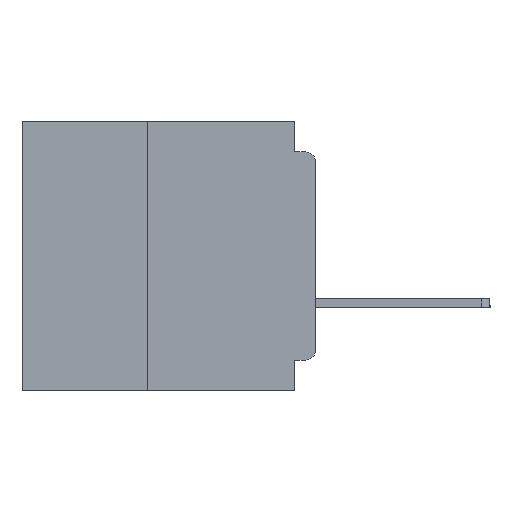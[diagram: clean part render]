
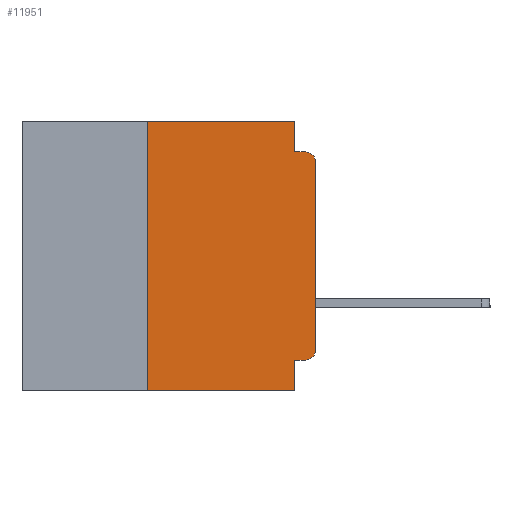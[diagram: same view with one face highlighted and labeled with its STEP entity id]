
A CAD part, left-side view. The second image highlights one B-rep face of the part: STEP entity #11951.
In plain terms, the highlighted planar face has unit normal (-1, 0, 0).
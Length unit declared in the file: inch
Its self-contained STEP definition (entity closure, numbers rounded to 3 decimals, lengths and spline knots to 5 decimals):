
#849 = PLANE ( 'NONE',  #15594 ) ;
#1895 = VERTEX_POINT ( 'NONE', #27323 ) ;
#2521 = ORIENTED_EDGE ( 'NONE', *, *, #34587, .F. ) ;
#2695 = LINE ( 'NONE', #43470, #38850 ) ;
#3022 = CARTESIAN_POINT ( 'NONE',  ( 0., 0.437, 0. ) ) ;
#3122 = EDGE_CURVE ( 'NONE', #5375, #38927, #2695, .T. ) ;
#3752 = ORIENTED_EDGE ( 'NONE', *, *, #7106, .F. ) ;
#3895 = CARTESIAN_POINT ( 'NONE',  ( 0., 0.25, -0.4 ) ) ;
#4044 = DIRECTION ( 'NONE',  ( 0., -1., 0. ) ) ;
#4057 = VERTEX_POINT ( 'NONE', #22687 ) ;
#4063 = DIRECTION ( 'NONE',  ( 0., -1., 0. ) ) ;
#4411 = DIRECTION ( 'NONE',  ( 0., 0., -1. ) ) ;
#5375 = VERTEX_POINT ( 'NONE', #37397 ) ;
#6188 = VECTOR ( 'NONE', #28904, 39.37008 ) ;
#6749 = CIRCLE ( 'NONE', #36059, 0.015 ) ;
#7106 = EDGE_CURVE ( 'NONE', #23628, #21815, #37991, .T. ) ;
#7167 = VERTEX_POINT ( 'NONE', #45107 ) ;
#7327 = LINE ( 'NONE', #12676, #25945 ) ;
#7833 = ORIENTED_EDGE ( 'NONE', *, *, #34651, .T. ) ;
#9080 = VECTOR ( 'NONE', #4044, 39.37008 ) ;
#9182 = DIRECTION ( 'NONE',  ( 0., 0., -1. ) ) ;
#9560 = CARTESIAN_POINT ( 'NONE',  ( 0., 0.015, -0.06 ) ) ;
#10347 = VECTOR ( 'NONE', #4063, 39.37008 ) ;
#10363 = EDGE_CURVE ( 'NONE', #4057, #17321, #6749, .T. ) ;
#11951 = ADVANCED_FACE ( 'NONE', ( #30230 ), #849, .F. ) ;
#12000 = ORIENTED_EDGE ( 'NONE', *, *, #3122, .T. ) ;
#12676 = CARTESIAN_POINT ( 'NONE',  ( 0., 0.031, 0. ) ) ;
#13090 = DIRECTION ( 'NONE',  ( 0., 0., -1. ) ) ;
#14006 = EDGE_LOOP ( 'NONE', ( #31859, #15687, #16194, #30568, #3752, #31439, #12000, #2521, #17823, #7833 ) ) ;
#14984 = EDGE_CURVE ( 'NONE', #5375, #23628, #25626, .T. ) ;
#15255 = VECTOR ( 'NONE', #31959, 39.37008 ) ;
#15594 = AXIS2_PLACEMENT_3D ( 'NONE', #39101, #25416, #4411 ) ;
#15687 = ORIENTED_EDGE ( 'NONE', *, *, #10363, .T. ) ;
#16194 = ORIENTED_EDGE ( 'NONE', *, *, #37518, .F. ) ;
#16230 = VERTEX_POINT ( 'NONE', #18100 ) ;
#16676 = DIRECTION ( 'NONE',  ( -1., 0., 0. ) ) ;
#17307 = EDGE_CURVE ( 'NONE', #21815, #7167, #7327, .T. ) ;
#17321 = VERTEX_POINT ( 'NONE', #33741 ) ;
#17823 = ORIENTED_EDGE ( 'NONE', *, *, #33784, .F. ) ;
#18100 = CARTESIAN_POINT ( 'NONE',  ( 0., 0., -0.34 ) ) ;
#21542 = CARTESIAN_POINT ( 'NONE',  ( 0., 0., -0.045 ) ) ;
#21815 = VERTEX_POINT ( 'NONE', #40271 ) ;
#22687 = CARTESIAN_POINT ( 'NONE',  ( 0., 0., -0.06 ) ) ;
#23628 = VERTEX_POINT ( 'NONE', #34811 ) ;
#25416 = DIRECTION ( 'NONE',  ( 1., 0., 0. ) ) ;
#25626 = LINE ( 'NONE', #3895, #15255 ) ;
#25945 = VECTOR ( 'NONE', #33581, 39.37008 ) ;
#26670 = CARTESIAN_POINT ( 'NONE',  ( 0., 0.031, -0.4 ) ) ;
#27323 = CARTESIAN_POINT ( 'NONE',  ( 0., 0.015, -0.355 ) ) ;
#27741 = LINE ( 'NONE', #44395, #37006 ) ;
#28904 = DIRECTION ( 'NONE',  ( 0., 1., 0. ) ) ;
#29144 = VECTOR ( 'NONE', #9182, 39.37008 ) ;
#29914 = VERTEX_POINT ( 'NONE', #36971 ) ;
#30230 = FACE_OUTER_BOUND ( 'NONE', #14006, .T. ) ;
#30568 = ORIENTED_EDGE ( 'NONE', *, *, #17307, .F. ) ;
#31439 = ORIENTED_EDGE ( 'NONE', *, *, #14984, .F. ) ;
#31859 = ORIENTED_EDGE ( 'NONE', *, *, #38977, .T. ) ;
#31959 = DIRECTION ( 'NONE',  ( 0., 0., 1. ) ) ;
#32396 = CARTESIAN_POINT ( 'NONE',  ( 0., 0., -0.355 ) ) ;
#33581 = DIRECTION ( 'NONE',  ( 0., 0., -1. ) ) ;
#33637 = CARTESIAN_POINT ( 'NONE',  ( 0., 0.031, -0.4 ) ) ;
#33741 = CARTESIAN_POINT ( 'NONE',  ( 0., 0.015, -0.045 ) ) ;
#33784 = EDGE_CURVE ( 'NONE', #1895, #29914, #43298, .T. ) ;
#34018 = DIRECTION ( 'NONE',  ( -1., 0., 0. ) ) ;
#34587 = EDGE_CURVE ( 'NONE', #29914, #38927, #39444, .T. ) ;
#34651 = EDGE_CURVE ( 'NONE', #1895, #16230, #35140, .T. ) ;
#34811 = CARTESIAN_POINT ( 'NONE',  ( 0., 0.25, 0. ) ) ;
#34934 = LINE ( 'NONE', #21542, #10347 ) ;
#35140 = CIRCLE ( 'NONE', #44611, 0.015 ) ;
#36059 = AXIS2_PLACEMENT_3D ( 'NONE', #9560, #34018, #13090 ) ;
#36971 = CARTESIAN_POINT ( 'NONE',  ( 0., 0.031, -0.355 ) ) ;
#37006 = VECTOR ( 'NONE', #44249, 39.37008 ) ;
#37397 = CARTESIAN_POINT ( 'NONE',  ( 0., 0.25, -0.4 ) ) ;
#37518 = EDGE_CURVE ( 'NONE', #7167, #17321, #34934, .T. ) ;
#37528 = CARTESIAN_POINT ( 'NONE',  ( 0., 0.015, -0.34 ) ) ;
#37991 = LINE ( 'NONE', #3022, #9080 ) ;
#38850 = VECTOR ( 'NONE', #43525, 39.37008 ) ;
#38927 = VERTEX_POINT ( 'NONE', #26670 ) ;
#38977 = EDGE_CURVE ( 'NONE', #16230, #4057, #27741, .T. ) ;
#39101 = CARTESIAN_POINT ( 'NONE',  ( 0., 0.437, 0. ) ) ;
#39444 = LINE ( 'NONE', #33637, #29144 ) ;
#40271 = CARTESIAN_POINT ( 'NONE',  ( 0., 0.031, 0. ) ) ;
#41022 = DIRECTION ( 'NONE',  ( 0., 0., -1. ) ) ;
#43298 = LINE ( 'NONE', #32396, #6188 ) ;
#43470 = CARTESIAN_POINT ( 'NONE',  ( 0., 0.437, -0.4 ) ) ;
#43525 = DIRECTION ( 'NONE',  ( 0., -1., 0. ) ) ;
#44249 = DIRECTION ( 'NONE',  ( 0., 0., 1. ) ) ;
#44395 = CARTESIAN_POINT ( 'NONE',  ( 0., 0., 0. ) ) ;
#44611 = AXIS2_PLACEMENT_3D ( 'NONE', #37528, #16676, #41022 ) ;
#45107 = CARTESIAN_POINT ( 'NONE',  ( 0., 0.031, -0.045 ) ) ;
